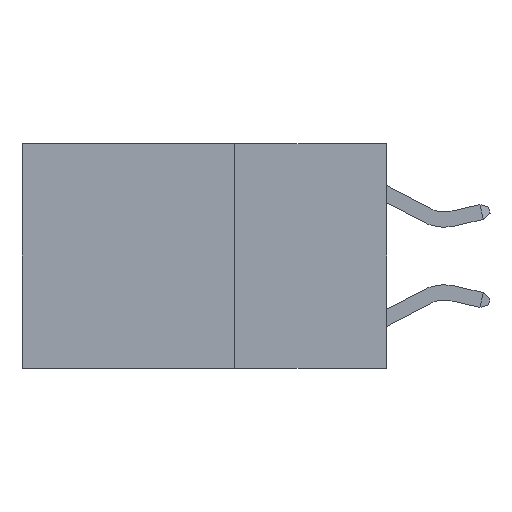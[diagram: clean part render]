
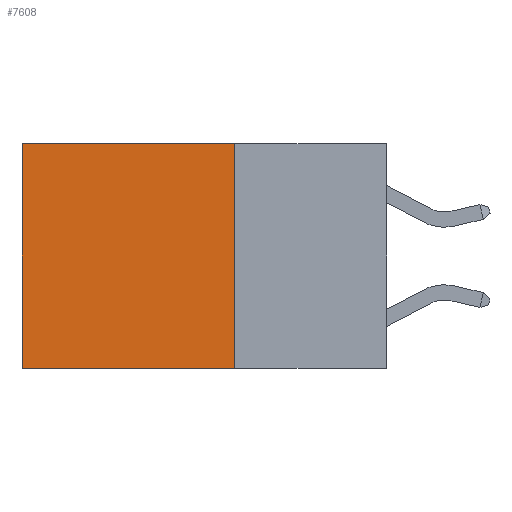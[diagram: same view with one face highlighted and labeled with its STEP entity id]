
A CAD part, left-side view. The second image highlights one B-rep face of the part: STEP entity #7608.
In plain terms, the highlighted planar face has unit normal (-1, 0, 0).
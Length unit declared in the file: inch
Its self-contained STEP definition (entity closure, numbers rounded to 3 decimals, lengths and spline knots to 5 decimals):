
#560 = VECTOR ( 'NONE', #11441, 39.37008 ) ;
#594 = CARTESIAN_POINT ( 'NONE',  ( 0.2625, 0.25, -0.37 ) ) ;
#641 = FACE_OUTER_BOUND ( 'NONE', #14464, .T. ) ;
#1559 = EDGE_CURVE ( 'NONE', #10557, #3647, #2647, .T. ) ;
#1585 = VERTEX_POINT ( 'NONE', #7766 ) ;
#1934 = CARTESIAN_POINT ( 'NONE',  ( 0.2625, 0.25, 0. ) ) ;
#2013 = LINE ( 'NONE', #10497, #560 ) ;
#2055 = DIRECTION ( 'NONE',  ( 0., 0., -1. ) ) ;
#2218 = ORIENTED_EDGE ( 'NONE', *, *, #6356, .T. ) ;
#2499 = VECTOR ( 'NONE', #9359, 39.37008 ) ;
#2647 = LINE ( 'NONE', #14866, #15161 ) ;
#3123 = EDGE_CURVE ( 'NONE', #3647, #13703, #9414, .T. ) ;
#3354 = CARTESIAN_POINT ( 'NONE',  ( 0.2625, 0.25, 0. ) ) ;
#3647 = VERTEX_POINT ( 'NONE', #594 ) ;
#4398 = EDGE_CURVE ( 'NONE', #1585, #13703, #2013, .T. ) ;
#4789 = VECTOR ( 'NONE', #7651, 39.37008 ) ;
#5751 = CARTESIAN_POINT ( 'NONE',  ( 0.2625, 0.6, -0.37 ) ) ;
#5752 = DIRECTION ( 'NONE',  ( 0., 0., -1. ) ) ;
#6260 = CARTESIAN_POINT ( 'NONE',  ( 0.2625, 0.25, 0. ) ) ;
#6356 = EDGE_CURVE ( 'NONE', #10557, #1585, #11680, .T. ) ;
#6518 = AXIS2_PLACEMENT_3D ( 'NONE', #3354, #11487, #2055 ) ;
#6912 = ORIENTED_EDGE ( 'NONE', *, *, #1559, .F. ) ;
#7608 = ADVANCED_FACE ( 'NONE', ( #641 ), #9191, .F. ) ;
#7651 = DIRECTION ( 'NONE',  ( 0., 1., 0. ) ) ;
#7766 = CARTESIAN_POINT ( 'NONE',  ( 0.2625, 0.6, 0. ) ) ;
#8783 = ORIENTED_EDGE ( 'NONE', *, *, #3123, .F. ) ;
#9191 = PLANE ( 'NONE',  #6518 ) ;
#9359 = DIRECTION ( 'NONE',  ( 0., 1., 0. ) ) ;
#9414 = LINE ( 'NONE', #12149, #4789 ) ;
#10497 = CARTESIAN_POINT ( 'NONE',  ( 0.2625, 0.6, 0. ) ) ;
#10557 = VERTEX_POINT ( 'NONE', #6260 ) ;
#11441 = DIRECTION ( 'NONE',  ( 0., 0., -1. ) ) ;
#11487 = DIRECTION ( 'NONE',  ( 1., 0., 0. ) ) ;
#11680 = LINE ( 'NONE', #1934, #2499 ) ;
#12149 = CARTESIAN_POINT ( 'NONE',  ( 0.2625, 0.25, -0.37 ) ) ;
#13242 = ORIENTED_EDGE ( 'NONE', *, *, #4398, .T. ) ;
#13703 = VERTEX_POINT ( 'NONE', #5751 ) ;
#14464 = EDGE_LOOP ( 'NONE', ( #13242, #8783, #6912, #2218 ) ) ;
#14866 = CARTESIAN_POINT ( 'NONE',  ( 0.2625, 0.25, 0. ) ) ;
#15161 = VECTOR ( 'NONE', #5752, 39.37008 ) ;
